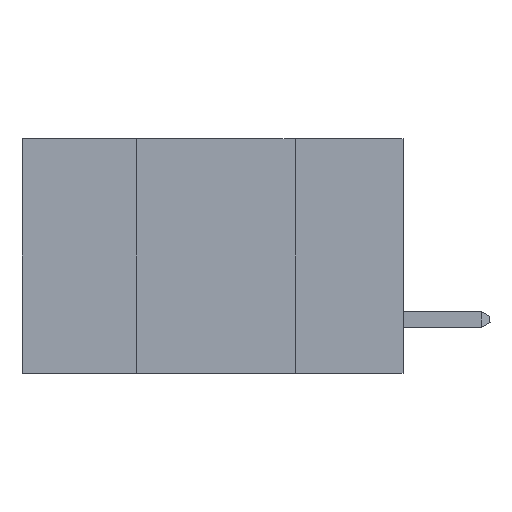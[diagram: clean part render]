
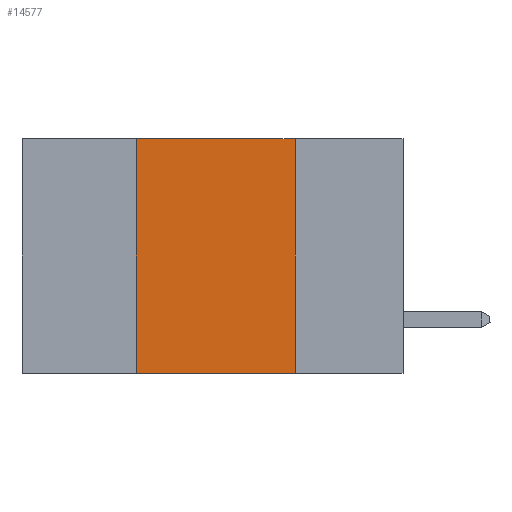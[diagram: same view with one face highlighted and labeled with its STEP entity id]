
A CAD part, left-side view. The second image highlights one B-rep face of the part: STEP entity #14577.
In plain terms, the highlighted planar face has unit normal (-1, 0, 0).
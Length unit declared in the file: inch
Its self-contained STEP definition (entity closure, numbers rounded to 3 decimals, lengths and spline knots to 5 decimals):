
#572 = LINE ( 'NONE', #3145, #18517 ) ;
#1383 = VERTEX_POINT ( 'NONE', #19491 ) ;
#1447 = VECTOR ( 'NONE', #2610, 39.37008 ) ;
#1956 = CARTESIAN_POINT ( 'NONE',  ( 0., 0.17, 0. ) ) ;
#2380 = ORIENTED_EDGE ( 'NONE', *, *, #21390, .T. ) ;
#2610 = DIRECTION ( 'NONE',  ( 0., -1., 0. ) ) ;
#3145 = CARTESIAN_POINT ( 'NONE',  ( 0., 0.42, 0. ) ) ;
#3538 = VECTOR ( 'NONE', #13934, 39.37008 ) ;
#4472 = VECTOR ( 'NONE', #22508, 39.37008 ) ;
#4481 = VERTEX_POINT ( 'NONE', #1956 ) ;
#6489 = FACE_OUTER_BOUND ( 'NONE', #22401, .T. ) ;
#6529 = ORIENTED_EDGE ( 'NONE', *, *, #9341, .F. ) ;
#7012 = VERTEX_POINT ( 'NONE', #10875 ) ;
#9272 = PLANE ( 'NONE',  #22162 ) ;
#9341 = EDGE_CURVE ( 'NONE', #7012, #11987, #572, .T. ) ;
#10875 = CARTESIAN_POINT ( 'NONE',  ( 0., 0.42, -0.37 ) ) ;
#11803 = EDGE_CURVE ( 'NONE', #11987, #4481, #15856, .T. ) ;
#11987 = VERTEX_POINT ( 'NONE', #22140 ) ;
#12570 = ORIENTED_EDGE ( 'NONE', *, *, #11803, .F. ) ;
#13663 = LINE ( 'NONE', #22416, #3538 ) ;
#13755 = ORIENTED_EDGE ( 'NONE', *, *, #17048, .F. ) ;
#13934 = DIRECTION ( 'NONE',  ( 0., 0., -1. ) ) ;
#14577 = ADVANCED_FACE ( 'NONE', ( #6489 ), #9272, .F. ) ;
#14579 = LINE ( 'NONE', #19837, #4472 ) ;
#15856 = LINE ( 'NONE', #19965, #1447 ) ;
#17048 = EDGE_CURVE ( 'NONE', #4481, #1383, #13663, .T. ) ;
#18517 = VECTOR ( 'NONE', #20008, 39.37008 ) ;
#19491 = CARTESIAN_POINT ( 'NONE',  ( 0., 0.17, -0.37 ) ) ;
#19837 = CARTESIAN_POINT ( 'NONE',  ( 0., 0.6, -0.37 ) ) ;
#19965 = CARTESIAN_POINT ( 'NONE',  ( 0., 0.6, 0. ) ) ;
#20008 = DIRECTION ( 'NONE',  ( 0., 0., 1. ) ) ;
#21273 = DIRECTION ( 'NONE',  ( 1., 0., 0. ) ) ;
#21390 = EDGE_CURVE ( 'NONE', #7012, #1383, #14579, .T. ) ;
#21419 = CARTESIAN_POINT ( 'NONE',  ( 0., 0.6, 0. ) ) ;
#21645 = DIRECTION ( 'NONE',  ( 0., 0., -1. ) ) ;
#22140 = CARTESIAN_POINT ( 'NONE',  ( 0., 0.42, 0. ) ) ;
#22162 = AXIS2_PLACEMENT_3D ( 'NONE', #21419, #21273, #21645 ) ;
#22401 = EDGE_LOOP ( 'NONE', ( #13755, #12570, #6529, #2380 ) ) ;
#22416 = CARTESIAN_POINT ( 'NONE',  ( 0., 0.17, 0. ) ) ;
#22508 = DIRECTION ( 'NONE',  ( 0., -1., 0. ) ) ;
